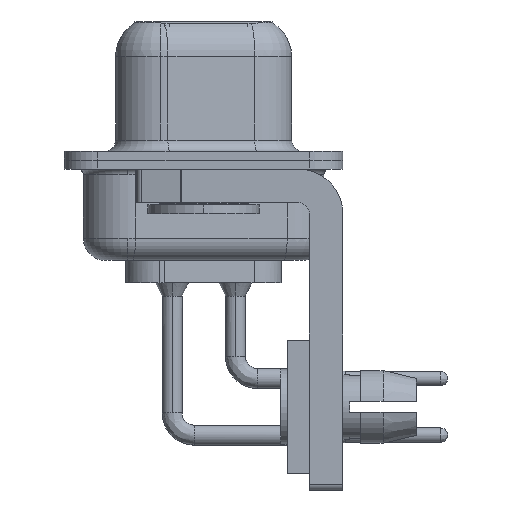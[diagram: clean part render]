
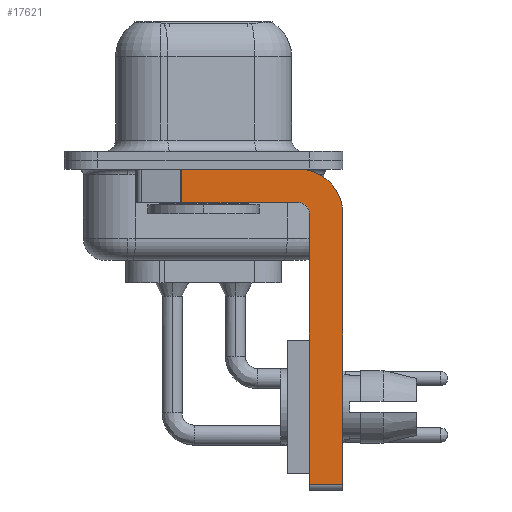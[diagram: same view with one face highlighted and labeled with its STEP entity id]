
A CAD part, left-side view. The second image highlights one B-rep face of the part: STEP entity #17621.
In plain terms, the highlighted planar face has unit normal (-1, 0, 0).
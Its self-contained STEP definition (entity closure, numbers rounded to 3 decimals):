
#432 = AXIS2_PLACEMENT_3D ( 'NONE', #3254, #23903, #11589 ) ;
#960 = ORIENTED_EDGE ( 'NONE', *, *, #1371, .F. ) ;
#1371 = EDGE_CURVE ( 'NONE', #18915, #3132, #4692, .T. ) ;
#1471 = LINE ( 'NONE', #11836, #22734 ) ;
#2248 = AXIS2_PLACEMENT_3D ( 'NONE', #4055, #18489, #6148 ) ;
#2251 = CARTESIAN_POINT ( 'NONE',  ( -2.9, -4.25, -2.4 ) ) ;
#2275 = LINE ( 'NONE', #5432, #6459 ) ;
#2704 = CARTESIAN_POINT ( 'NONE',  ( -2.9, -4.75, -14.55 ) ) ;
#3132 = VERTEX_POINT ( 'NONE', #11948 ) ;
#3254 = CARTESIAN_POINT ( 'NONE',  ( -2.9, -4.25, -2.4 ) ) ;
#3309 = VERTEX_POINT ( 'NONE', #13986 ) ;
#3550 = CARTESIAN_POINT ( 'NONE',  ( -2.9, 0.978, -1.9 ) ) ;
#3796 = VECTOR ( 'NONE', #24519, 1000. ) ;
#4055 = CARTESIAN_POINT ( 'NONE',  ( -2.9, -4.25, -2.4 ) ) ;
#4307 = DIRECTION ( 'NONE',  ( 0., 0., -1. ) ) ;
#4692 = LINE ( 'NONE', #15050, #26605 ) ;
#5138 = EDGE_CURVE ( 'NONE', #18915, #20252, #2275, .T. ) ;
#5316 = EDGE_CURVE ( 'NONE', #3132, #9706, #14205, .T. ) ;
#5336 = PLANE ( 'NONE',  #432 ) ;
#5432 = CARTESIAN_POINT ( 'NONE',  ( -2.9, -4.25, -14.55 ) ) ;
#5517 = CARTESIAN_POINT ( 'NONE',  ( -2.9, -6.25, -14.55 ) ) ;
#5526 = DIRECTION ( 'NONE',  ( 0., -1., 0. ) ) ;
#5758 = DIRECTION ( 'NONE',  ( 0., -1., 0. ) ) ;
#5895 = EDGE_CURVE ( 'NONE', #17464, #3309, #17703, .T. ) ;
#6148 = DIRECTION ( 'NONE',  ( 0., 0., 1. ) ) ;
#6302 = VERTEX_POINT ( 'NONE', #3550 ) ;
#6459 = VECTOR ( 'NONE', #5526, 1000. ) ;
#7106 = EDGE_CURVE ( 'NONE', #3309, #20252, #9972, .T. ) ;
#9188 = LINE ( 'NONE', #22227, #18834 ) ;
#9538 = EDGE_LOOP ( 'NONE', ( #15700, #13838, #25416, #24460, #960, #13554, #13246, #10285 ) ) ;
#9706 = VERTEX_POINT ( 'NONE', #24208 ) ;
#9972 = LINE ( 'NONE', #18307, #3796 ) ;
#10285 = ORIENTED_EDGE ( 'NONE', *, *, #5895, .F. ) ;
#11589 = DIRECTION ( 'NONE',  ( 0., 0., -1. ) ) ;
#11836 = CARTESIAN_POINT ( 'NONE',  ( -2.9, 0.978, -1.9 ) ) ;
#11948 = CARTESIAN_POINT ( 'NONE',  ( -2.9, -4.75, -2.4 ) ) ;
#13246 = ORIENTED_EDGE ( 'NONE', *, *, #7106, .F. ) ;
#13554 = ORIENTED_EDGE ( 'NONE', *, *, #5138, .T. ) ;
#13838 = ORIENTED_EDGE ( 'NONE', *, *, #24798, .T. ) ;
#13842 = DIRECTION ( 'NONE',  ( 0., 1., 0. ) ) ;
#13986 = CARTESIAN_POINT ( 'NONE',  ( -2.9, -6.25, -2.4 ) ) ;
#14105 = CARTESIAN_POINT ( 'NONE',  ( -2.9, 0.978, -0.4 ) ) ;
#14205 = CIRCLE ( 'NONE', #2248, 0.5 ) ;
#14283 = EDGE_CURVE ( 'NONE', #14974, #17464, #9188, .T. ) ;
#14878 = EDGE_CURVE ( 'NONE', #9706, #6302, #20282, .T. ) ;
#14974 = VERTEX_POINT ( 'NONE', #14105 ) ;
#15050 = CARTESIAN_POINT ( 'NONE',  ( -2.9, -4.75, -14.8 ) ) ;
#15700 = ORIENTED_EDGE ( 'NONE', *, *, #14283, .F. ) ;
#16433 = AXIS2_PLACEMENT_3D ( 'NONE', #2251, #16680, #4307 ) ;
#16680 = DIRECTION ( 'NONE',  ( 1., 0., 0. ) ) ;
#17464 = VERTEX_POINT ( 'NONE', #23272 ) ;
#17621 = ADVANCED_FACE ( 'NONE', ( #20523 ), #5336, .F. ) ;
#17703 = CIRCLE ( 'NONE', #16433, 2. ) ;
#18307 = CARTESIAN_POINT ( 'NONE',  ( -2.9, -6.25, -2.4 ) ) ;
#18400 = DIRECTION ( 'NONE',  ( 0., 0., 1. ) ) ;
#18489 = DIRECTION ( 'NONE',  ( -1., 0., 0. ) ) ;
#18834 = VECTOR ( 'NONE', #5758, 1000. ) ;
#18915 = VERTEX_POINT ( 'NONE', #2704 ) ;
#19009 = VECTOR ( 'NONE', #13842, 1000. ) ;
#20252 = VERTEX_POINT ( 'NONE', #5517 ) ;
#20282 = LINE ( 'NONE', #24096, #19009 ) ;
#20523 = FACE_OUTER_BOUND ( 'NONE', #9538, .T. ) ;
#22227 = CARTESIAN_POINT ( 'NONE',  ( -2.9, 3., -0.4 ) ) ;
#22734 = VECTOR ( 'NONE', #24140, 1000. ) ;
#23272 = CARTESIAN_POINT ( 'NONE',  ( -2.9, -4.25, -0.4 ) ) ;
#23903 = DIRECTION ( 'NONE',  ( 1., 0., 0. ) ) ;
#24096 = CARTESIAN_POINT ( 'NONE',  ( -2.9, -4.25, -1.9 ) ) ;
#24140 = DIRECTION ( 'NONE',  ( 0., 0., -1. ) ) ;
#24208 = CARTESIAN_POINT ( 'NONE',  ( -2.9, -4.25, -1.9 ) ) ;
#24460 = ORIENTED_EDGE ( 'NONE', *, *, #5316, .F. ) ;
#24519 = DIRECTION ( 'NONE',  ( 0., 0., -1. ) ) ;
#24798 = EDGE_CURVE ( 'NONE', #14974, #6302, #1471, .T. ) ;
#25416 = ORIENTED_EDGE ( 'NONE', *, *, #14878, .F. ) ;
#26605 = VECTOR ( 'NONE', #18400, 1000. ) ;
